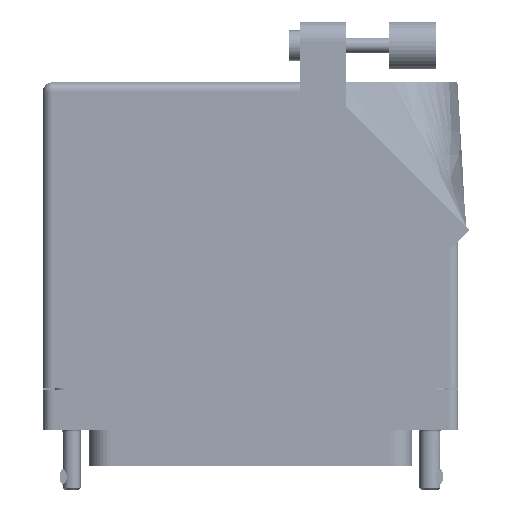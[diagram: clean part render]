
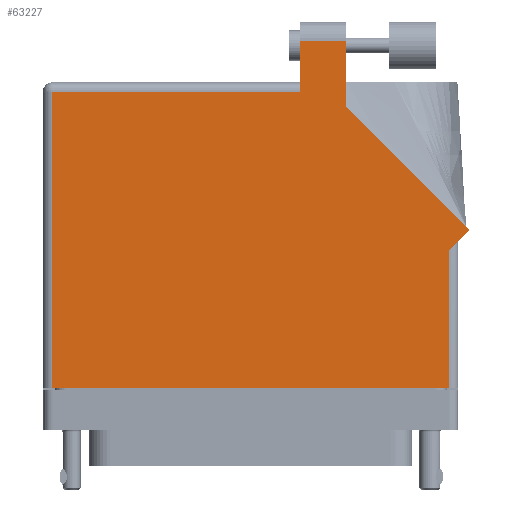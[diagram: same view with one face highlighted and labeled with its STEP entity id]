
A CAD part, front view. The second image highlights one B-rep face of the part: STEP entity #63227.
In plain terms, the highlighted face is planar.
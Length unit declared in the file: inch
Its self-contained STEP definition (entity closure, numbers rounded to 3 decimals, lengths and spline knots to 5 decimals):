
#1863 = EDGE_CURVE ( 'NONE', #78288, #17381, #82338, .T. ) ;
#2753 = CARTESIAN_POINT ( 'NONE',  ( 0.6345, 1.76442, 0.765 ) ) ;
#3000 = VECTOR ( 'NONE', #13855, 39.37008 ) ;
#3486 = ORIENTED_EDGE ( 'NONE', *, *, #23408, .T. ) ;
#4686 = FACE_OUTER_BOUND ( 'NONE', #77350, .T. ) ;
#5654 = ORIENTED_EDGE ( 'NONE', *, *, #102342, .T. ) ;
#6380 = CARTESIAN_POINT ( 'NONE',  ( -1.3155, -0.1, 0.765 ) ) ;
#9573 = DIRECTION ( 'NONE',  ( -0.707, 0.707, 0. ) ) ;
#9795 = CARTESIAN_POINT ( 'NONE',  ( 0.6345, 2.205, 0.765 ) ) ;
#12309 = CARTESIAN_POINT ( 'NONE',  ( 0.3275, 1.868, 0.765 ) ) ;
#13855 = DIRECTION ( 'NONE',  ( 0.707, 0.707, 0. ) ) ;
#14191 = ORIENTED_EDGE ( 'NONE', *, *, #51603, .T. ) ;
#16555 = LINE ( 'NONE', #47497, #36373 ) ;
#17381 = VERTEX_POINT ( 'NONE', #12309 ) ;
#18212 = CARTESIAN_POINT ( 'NONE',  ( 1.44821, 0.95071, 0.765 ) ) ;
#21207 = CARTESIAN_POINT ( 'NONE',  ( 0.3275, 2.205, 0.765 ) ) ;
#21531 = CARTESIAN_POINT ( 'NONE',  ( 0.3275, 2.205, 0.765 ) ) ;
#23088 = EDGE_CURVE ( 'NONE', #72708, #60104, #61298, .T. ) ;
#23408 = EDGE_CURVE ( 'NONE', #52149, #57207, #83723, .T. ) ;
#23898 = CARTESIAN_POINT ( 'NONE',  ( 1.3155, -0.1, 0.765 ) ) ;
#24531 = DIRECTION ( 'NONE',  ( 0., 1., 0. ) ) ;
#24903 = CARTESIAN_POINT ( 'NONE',  ( 0.3275, 1.93, 0.765 ) ) ;
#28275 = VECTOR ( 'NONE', #93308, 39.37008 ) ;
#30281 = DIRECTION ( 'NONE',  ( -1., 0., 0. ) ) ;
#34162 = EDGE_CURVE ( 'NONE', #91721, #45217, #16555, .T. ) ;
#35558 = VECTOR ( 'NONE', #66969, 39.37008 ) ;
#36373 = VECTOR ( 'NONE', #79223, 39.37008 ) ;
#36524 = ORIENTED_EDGE ( 'NONE', *, *, #34162, .T. ) ;
#36811 = PLANE ( 'NONE',  #48223 ) ;
#37616 = VECTOR ( 'NONE', #9573, 39.37008 ) ;
#37690 = LINE ( 'NONE', #78182, #3000 ) ;
#38620 = LINE ( 'NONE', #21531, #53622 ) ;
#45217 = VERTEX_POINT ( 'NONE', #6380 ) ;
#46192 = DIRECTION ( 'NONE',  ( 0., 0., -1. ) ) ;
#47497 = CARTESIAN_POINT ( 'NONE',  ( -1.3155, -0.1, 0.765 ) ) ;
#48223 = AXIS2_PLACEMENT_3D ( 'NONE', #54149, #46192, #30281 ) ;
#48554 = ORIENTED_EDGE ( 'NONE', *, *, #66130, .T. ) ;
#51100 = VECTOR ( 'NONE', #64825, 39.37008 ) ;
#51603 = EDGE_CURVE ( 'NONE', #17381, #91721, #69369, .T. ) ;
#52149 = VERTEX_POINT ( 'NONE', #23898 ) ;
#52250 = VECTOR ( 'NONE', #70725, 39.37008 ) ;
#53622 = VECTOR ( 'NONE', #62809, 39.37008 ) ;
#54149 = CARTESIAN_POINT ( 'NONE',  ( -1.3775, 1.93, 0.765 ) ) ;
#55361 = LINE ( 'NONE', #2753, #35558 ) ;
#57207 = VERTEX_POINT ( 'NONE', #83879 ) ;
#58614 = EDGE_CURVE ( 'NONE', #60556, #78288, #38620, .T. ) ;
#60104 = VERTEX_POINT ( 'NONE', #73062 ) ;
#60556 = VERTEX_POINT ( 'NONE', #9795 ) ;
#61298 = LINE ( 'NONE', #71804, #37616 ) ;
#61514 = ORIENTED_EDGE ( 'NONE', *, *, #71153, .T. ) ;
#62403 = CARTESIAN_POINT ( 'NONE',  ( -1.3775, -0.1, 0.765 ) ) ;
#62519 = VECTOR ( 'NONE', #24531, 39.37008 ) ;
#62809 = DIRECTION ( 'NONE',  ( -1., 0., 0. ) ) ;
#63227 = ADVANCED_FACE ( 'NONE', ( #4686 ), #36811, .F. ) ;
#64825 = DIRECTION ( 'NONE',  ( 0., -1., 0. ) ) ;
#66130 = EDGE_CURVE ( 'NONE', #57207, #72708, #37690, .T. ) ;
#66969 = DIRECTION ( 'NONE',  ( 0., 1., 0. ) ) ;
#68468 = CARTESIAN_POINT ( 'NONE',  ( -1.3155, 1.868, 0.765 ) ) ;
#69369 = LINE ( 'NONE', #70605, #28275 ) ;
#70327 = ORIENTED_EDGE ( 'NONE', *, *, #23088, .T. ) ;
#70605 = CARTESIAN_POINT ( 'NONE',  ( -1.3775, 1.868, 0.765 ) ) ;
#70725 = DIRECTION ( 'NONE',  ( 1., 0., 0. ) ) ;
#71153 = EDGE_CURVE ( 'NONE', #60104, #60556, #55361, .T. ) ;
#71804 = CARTESIAN_POINT ( 'NONE',  ( 1.44821, 0.95071, 0.765 ) ) ;
#72708 = VERTEX_POINT ( 'NONE', #18212 ) ;
#73062 = CARTESIAN_POINT ( 'NONE',  ( 0.6345, 1.76442, 0.765 ) ) ;
#73145 = ORIENTED_EDGE ( 'NONE', *, *, #58614, .T. ) ;
#73460 = LINE ( 'NONE', #62403, #52250 ) ;
#75620 = ORIENTED_EDGE ( 'NONE', *, *, #1863, .T. ) ;
#77350 = EDGE_LOOP ( 'NONE', ( #61514, #73145, #75620, #14191, #36524, #5654, #3486, #48554, #70327 ) ) ;
#78182 = CARTESIAN_POINT ( 'NONE',  ( 1.3775, 0.88, 0.765 ) ) ;
#78288 = VERTEX_POINT ( 'NONE', #21207 ) ;
#79223 = DIRECTION ( 'NONE',  ( 0., -1., 0. ) ) ;
#82338 = LINE ( 'NONE', #24903, #51100 ) ;
#83723 = LINE ( 'NONE', #87520, #62519 ) ;
#83879 = CARTESIAN_POINT ( 'NONE',  ( 1.3155, 0.818, 0.765 ) ) ;
#87520 = CARTESIAN_POINT ( 'NONE',  ( 1.3155, 0.88, 0.765 ) ) ;
#91721 = VERTEX_POINT ( 'NONE', #68468 ) ;
#93308 = DIRECTION ( 'NONE',  ( -1., 0., 0. ) ) ;
#102342 = EDGE_CURVE ( 'NONE', #45217, #52149, #73460, .T. ) ;
